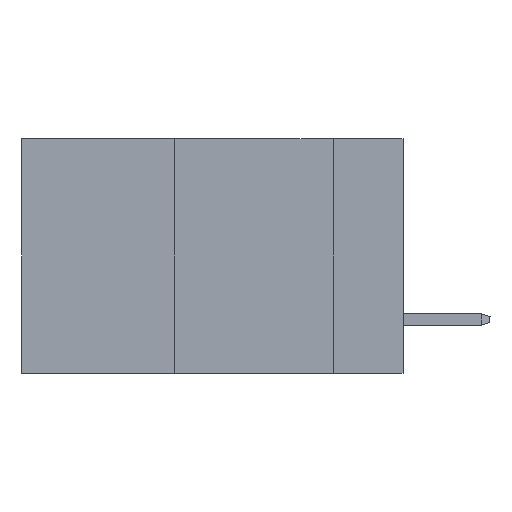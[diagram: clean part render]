
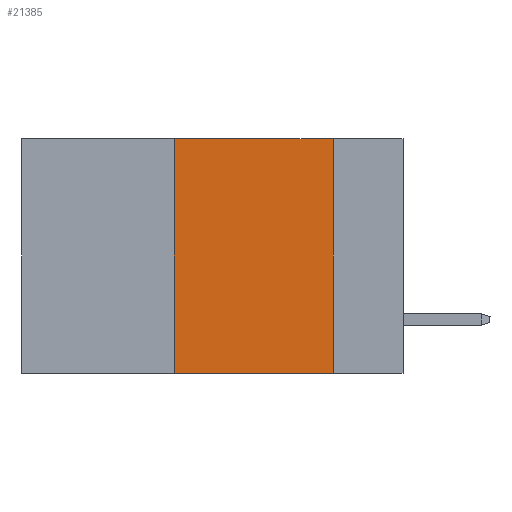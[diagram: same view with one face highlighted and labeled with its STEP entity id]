
A CAD part, left-side view. The second image highlights one B-rep face of the part: STEP entity #21385.
In plain terms, the highlighted planar face has unit normal (-1, 0, 0).
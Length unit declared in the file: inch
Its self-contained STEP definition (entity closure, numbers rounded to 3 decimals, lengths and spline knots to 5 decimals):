
#1600 = ORIENTED_EDGE ( 'NONE', *, *, #28083, .F. ) ;
#4577 = EDGE_CURVE ( 'NONE', #24899, #27179, #11423, .T. ) ;
#7646 = AXIS2_PLACEMENT_3D ( 'NONE', #17386, #34322, #20156 ) ;
#7867 = ORIENTED_EDGE ( 'NONE', *, *, #10358, .F. ) ;
#8062 = VECTOR ( 'NONE', #34201, 39.37008 ) ;
#10358 = EDGE_CURVE ( 'NONE', #14333, #27179, #22824, .T. ) ;
#11423 = LINE ( 'NONE', #22385, #31833 ) ;
#12219 = CARTESIAN_POINT ( 'NONE',  ( 0., 0.6, 0. ) ) ;
#13362 = CARTESIAN_POINT ( 'NONE',  ( 0., 0.36, 0. ) ) ;
#14333 = VERTEX_POINT ( 'NONE', #34949 ) ;
#17386 = CARTESIAN_POINT ( 'NONE',  ( 0., 0.6, 0. ) ) ;
#17469 = ORIENTED_EDGE ( 'NONE', *, *, #34927, .F. ) ;
#18484 = ORIENTED_EDGE ( 'NONE', *, *, #4577, .T. ) ;
#20156 = DIRECTION ( 'NONE',  ( 0., 0., -1. ) ) ;
#21385 = ADVANCED_FACE ( 'NONE', ( #22961 ), #34503, .F. ) ;
#22385 = CARTESIAN_POINT ( 'NONE',  ( 0., 0.6, -0.37 ) ) ;
#22746 = DIRECTION ( 'NONE',  ( 0., -1., 0. ) ) ;
#22824 = LINE ( 'NONE', #31395, #8062 ) ;
#22961 = FACE_OUTER_BOUND ( 'NONE', #33035, .T. ) ;
#24899 = VERTEX_POINT ( 'NONE', #26978 ) ;
#26906 = LINE ( 'NONE', #12219, #32773 ) ;
#26978 = CARTESIAN_POINT ( 'NONE',  ( 0., 0.36, -0.37 ) ) ;
#27179 = VERTEX_POINT ( 'NONE', #28846 ) ;
#28083 = EDGE_CURVE ( 'NONE', #24899, #29067, #29494, .T. ) ;
#28629 = VECTOR ( 'NONE', #35432, 39.37008 ) ;
#28846 = CARTESIAN_POINT ( 'NONE',  ( 0., 0.11, -0.37 ) ) ;
#29067 = VERTEX_POINT ( 'NONE', #13362 ) ;
#29494 = LINE ( 'NONE', #35075, #28629 ) ;
#31395 = CARTESIAN_POINT ( 'NONE',  ( 0., 0.11, 0. ) ) ;
#31833 = VECTOR ( 'NONE', #22746, 39.37008 ) ;
#32773 = VECTOR ( 'NONE', #32883, 39.37008 ) ;
#32883 = DIRECTION ( 'NONE',  ( 0., -1., 0. ) ) ;
#33035 = EDGE_LOOP ( 'NONE', ( #7867, #17469, #1600, #18484 ) ) ;
#34201 = DIRECTION ( 'NONE',  ( 0., 0., -1. ) ) ;
#34322 = DIRECTION ( 'NONE',  ( 1., 0., 0. ) ) ;
#34503 = PLANE ( 'NONE',  #7646 ) ;
#34927 = EDGE_CURVE ( 'NONE', #29067, #14333, #26906, .T. ) ;
#34949 = CARTESIAN_POINT ( 'NONE',  ( 0., 0.11, 0. ) ) ;
#35075 = CARTESIAN_POINT ( 'NONE',  ( 0., 0.36, 0. ) ) ;
#35432 = DIRECTION ( 'NONE',  ( 0., 0., 1. ) ) ;
